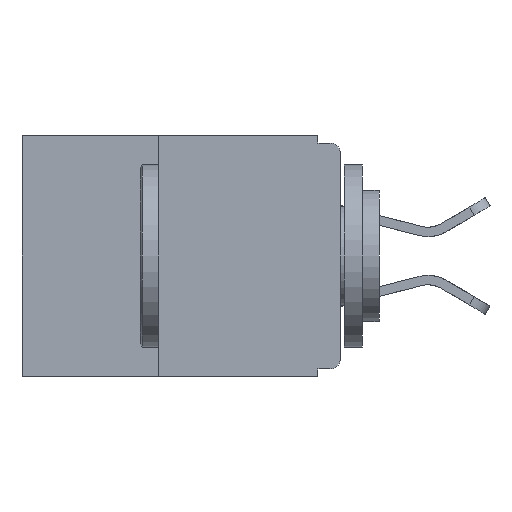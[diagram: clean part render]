
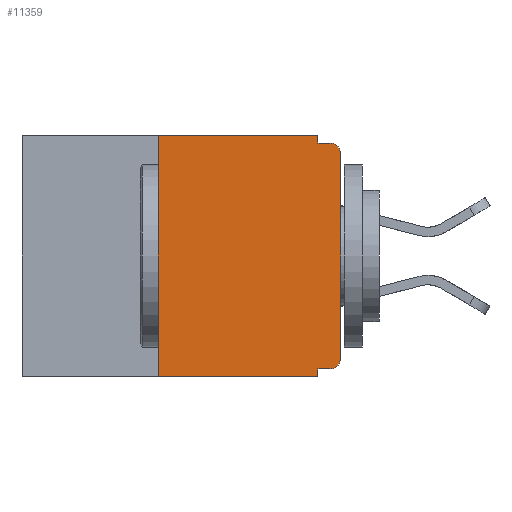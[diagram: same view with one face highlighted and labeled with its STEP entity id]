
A CAD part, left-side view. The second image highlights one B-rep face of the part: STEP entity #11359.
In plain terms, the highlighted planar face has unit normal (-1, 0, 0).
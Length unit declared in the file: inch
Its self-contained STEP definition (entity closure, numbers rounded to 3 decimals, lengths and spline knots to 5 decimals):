
#490 = CARTESIAN_POINT ( 'NONE',  ( 0., 0.437, -0.33 ) ) ;
#571 = EDGE_CURVE ( 'NONE', #16428, #21467, #18865, .T. ) ;
#779 = CARTESIAN_POINT ( 'NONE',  ( 0., 0., -0.025 ) ) ;
#898 = CARTESIAN_POINT ( 'NONE',  ( 0., 0.015, -0.305 ) ) ;
#1137 = LINE ( 'NONE', #490, #11105 ) ;
#1376 = FACE_OUTER_BOUND ( 'NONE', #17624, .T. ) ;
#1506 = DIRECTION ( 'NONE',  ( 0., 0., 1. ) ) ;
#1567 = CARTESIAN_POINT ( 'NONE',  ( 0., 0.25, -0.33 ) ) ;
#1582 = CARTESIAN_POINT ( 'NONE',  ( 0., 0.25, -0.33 ) ) ;
#1588 = EDGE_CURVE ( 'NONE', #13133, #15607, #1137, .T. ) ;
#1713 = CARTESIAN_POINT ( 'NONE',  ( 0., 0.015, -0.025 ) ) ;
#1822 = LINE ( 'NONE', #12108, #22811 ) ;
#2058 = LINE ( 'NONE', #1567, #23645 ) ;
#2659 = CARTESIAN_POINT ( 'NONE',  ( 0., 0.015, -0.32 ) ) ;
#2665 = CARTESIAN_POINT ( 'NONE',  ( 0., 0.015, -0.01 ) ) ;
#2853 = VECTOR ( 'NONE', #8718, 39.37008 ) ;
#2903 = LINE ( 'NONE', #21154, #23232 ) ;
#3146 = VECTOR ( 'NONE', #10557, 39.37008 ) ;
#3316 = CIRCLE ( 'NONE', #21995, 0.015 ) ;
#3592 = VERTEX_POINT ( 'NONE', #17115 ) ;
#3717 = DIRECTION ( 'NONE',  ( 0., 0., -1. ) ) ;
#3727 = DIRECTION ( 'NONE',  ( 0., 0., 1. ) ) ;
#3894 = EDGE_CURVE ( 'NONE', #3592, #24115, #1822, .T. ) ;
#4104 = CARTESIAN_POINT ( 'NONE',  ( 0., 0., 0. ) ) ;
#4261 = ORIENTED_EDGE ( 'NONE', *, *, #21170, .F. ) ;
#5133 = DIRECTION ( 'NONE',  ( 0., 0., -1. ) ) ;
#5353 = EDGE_CURVE ( 'NONE', #21467, #23357, #18504, .T. ) ;
#5417 = EDGE_CURVE ( 'NONE', #13133, #19260, #2058, .T. ) ;
#6207 = CARTESIAN_POINT ( 'NONE',  ( 0., 0.25, 0. ) ) ;
#6748 = CARTESIAN_POINT ( 'NONE',  ( 0., 0., -0.01 ) ) ;
#7266 = CARTESIAN_POINT ( 'NONE',  ( 0., 0.031, -0.32 ) ) ;
#7274 = AXIS2_PLACEMENT_3D ( 'NONE', #898, #13901, #5133 ) ;
#7356 = EDGE_CURVE ( 'NONE', #19260, #3592, #2903, .T. ) ;
#7934 = ORIENTED_EDGE ( 'NONE', *, *, #12877, .F. ) ;
#8718 = DIRECTION ( 'NONE',  ( 0., -1., 0. ) ) ;
#9186 = ORIENTED_EDGE ( 'NONE', *, *, #3894, .F. ) ;
#9853 = PLANE ( 'NONE',  #17279 ) ;
#10490 = ORIENTED_EDGE ( 'NONE', *, *, #1588, .T. ) ;
#10557 = DIRECTION ( 'NONE',  ( 0., 0., -1. ) ) ;
#11016 = CARTESIAN_POINT ( 'NONE',  ( 0., 0.031, -0.33 ) ) ;
#11105 = VECTOR ( 'NONE', #11133, 39.37008 ) ;
#11133 = DIRECTION ( 'NONE',  ( 0., -1., 0. ) ) ;
#11359 = ADVANCED_FACE ( 'NONE', ( #1376 ), #9853, .F. ) ;
#12108 = CARTESIAN_POINT ( 'NONE',  ( 0., 0.031, 0. ) ) ;
#12438 = DIRECTION ( 'NONE',  ( 0., 0., -1. ) ) ;
#12877 = EDGE_CURVE ( 'NONE', #24115, #24897, #13411, .T. ) ;
#12999 = CARTESIAN_POINT ( 'NONE',  ( 0., 0.031, -0.01 ) ) ;
#13133 = VERTEX_POINT ( 'NONE', #1582 ) ;
#13254 = VECTOR ( 'NONE', #3727, 39.37008 ) ;
#13411 = LINE ( 'NONE', #6748, #2853 ) ;
#13826 = DIRECTION ( 'NONE',  ( 0., 0., -1. ) ) ;
#13901 = DIRECTION ( 'NONE',  ( -1., 0., 0. ) ) ;
#15372 = DIRECTION ( 'NONE',  ( 1., 0., 0. ) ) ;
#15597 = DIRECTION ( 'NONE',  ( -1., 0., 0. ) ) ;
#15607 = VERTEX_POINT ( 'NONE', #11016 ) ;
#15996 = ORIENTED_EDGE ( 'NONE', *, *, #5353, .T. ) ;
#16049 = ORIENTED_EDGE ( 'NONE', *, *, #571, .T. ) ;
#16428 = VERTEX_POINT ( 'NONE', #2659 ) ;
#17115 = CARTESIAN_POINT ( 'NONE',  ( 0., 0.031, 0. ) ) ;
#17258 = ORIENTED_EDGE ( 'NONE', *, *, #21855, .T. ) ;
#17279 = AXIS2_PLACEMENT_3D ( 'NONE', #23565, #15372, #13826 ) ;
#17539 = CARTESIAN_POINT ( 'NONE',  ( 0., 0., -0.32 ) ) ;
#17624 = EDGE_LOOP ( 'NONE', ( #15996, #17258, #7934, #9186, #25406, #22712, #10490, #4261, #20024, #16049 ) ) ;
#17919 = VERTEX_POINT ( 'NONE', #7266 ) ;
#18108 = VECTOR ( 'NONE', #25293, 39.37008 ) ;
#18504 = LINE ( 'NONE', #4104, #13254 ) ;
#18865 = CIRCLE ( 'NONE', #7274, 0.015 ) ;
#19260 = VERTEX_POINT ( 'NONE', #6207 ) ;
#19712 = EDGE_CURVE ( 'NONE', #16428, #17919, #23249, .T. ) ;
#20024 = ORIENTED_EDGE ( 'NONE', *, *, #19712, .F. ) ;
#20340 = CARTESIAN_POINT ( 'NONE',  ( 0., 0.031, -0.33 ) ) ;
#21154 = CARTESIAN_POINT ( 'NONE',  ( 0., 0.437, 0. ) ) ;
#21170 = EDGE_CURVE ( 'NONE', #17919, #15607, #24082, .T. ) ;
#21467 = VERTEX_POINT ( 'NONE', #23110 ) ;
#21855 = EDGE_CURVE ( 'NONE', #23357, #24897, #3316, .T. ) ;
#21995 = AXIS2_PLACEMENT_3D ( 'NONE', #1713, #15597, #3717 ) ;
#22027 = DIRECTION ( 'NONE',  ( 0., -1., 0. ) ) ;
#22712 = ORIENTED_EDGE ( 'NONE', *, *, #5417, .F. ) ;
#22811 = VECTOR ( 'NONE', #12438, 39.37008 ) ;
#23110 = CARTESIAN_POINT ( 'NONE',  ( 0., 0., -0.305 ) ) ;
#23232 = VECTOR ( 'NONE', #22027, 39.37008 ) ;
#23249 = LINE ( 'NONE', #17539, #18108 ) ;
#23357 = VERTEX_POINT ( 'NONE', #779 ) ;
#23565 = CARTESIAN_POINT ( 'NONE',  ( 0., 0.437, 0. ) ) ;
#23645 = VECTOR ( 'NONE', #1506, 39.37008 ) ;
#24082 = LINE ( 'NONE', #20340, #3146 ) ;
#24115 = VERTEX_POINT ( 'NONE', #12999 ) ;
#24897 = VERTEX_POINT ( 'NONE', #2665 ) ;
#25293 = DIRECTION ( 'NONE',  ( 0., 1., 0. ) ) ;
#25406 = ORIENTED_EDGE ( 'NONE', *, *, #7356, .F. ) ;
